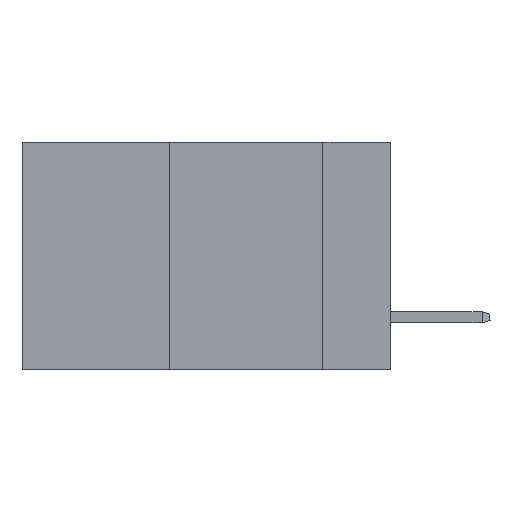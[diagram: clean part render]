
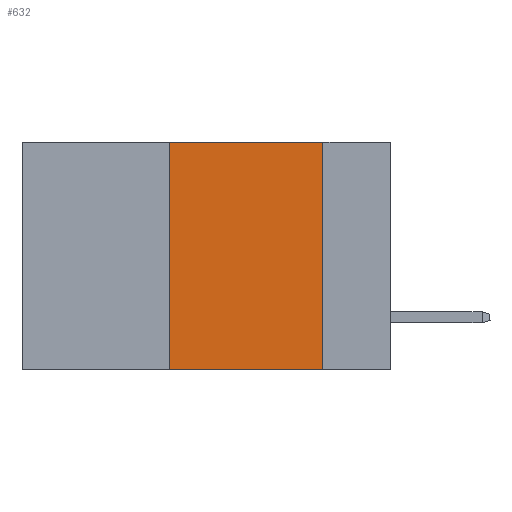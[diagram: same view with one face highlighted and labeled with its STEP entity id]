
A CAD part, left-side view. The second image highlights one B-rep face of the part: STEP entity #632.
In plain terms, the highlighted planar face has unit normal (-1, 0, 0).
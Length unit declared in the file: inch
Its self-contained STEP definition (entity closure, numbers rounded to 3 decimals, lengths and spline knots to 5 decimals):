
#632 = ADVANCED_FACE ( 'NONE', ( #15207 ), #27945, .F. ) ;
#951 = VECTOR ( 'NONE', #22163, 39.37008 ) ;
#1521 = CARTESIAN_POINT ( 'NONE',  ( 0., 0.36, -0.37 ) ) ;
#1534 = DIRECTION ( 'NONE',  ( 0., -1., 0. ) ) ;
#1696 = DIRECTION ( 'NONE',  ( 0., 0., -1. ) ) ;
#2200 = VERTEX_POINT ( 'NONE', #24171 ) ;
#4333 = ORIENTED_EDGE ( 'NONE', *, *, #21173, .F. ) ;
#4380 = LINE ( 'NONE', #22744, #18319 ) ;
#4994 = VERTEX_POINT ( 'NONE', #8363 ) ;
#7084 = LINE ( 'NONE', #18737, #25056 ) ;
#8363 = CARTESIAN_POINT ( 'NONE',  ( 0., 0.11, 0. ) ) ;
#8763 = LINE ( 'NONE', #22068, #951 ) ;
#9481 = EDGE_LOOP ( 'NONE', ( #4333, #19228, #18112, #19227 ) ) ;
#10338 = EDGE_CURVE ( 'NONE', #14017, #14317, #19107, .T. ) ;
#10437 = CARTESIAN_POINT ( 'NONE',  ( 0., 0.6, -0.37 ) ) ;
#12323 = DIRECTION ( 'NONE',  ( 0., -1., 0. ) ) ;
#14017 = VERTEX_POINT ( 'NONE', #1521 ) ;
#14317 = VERTEX_POINT ( 'NONE', #24452 ) ;
#14990 = DIRECTION ( 'NONE',  ( 1., 0., 0. ) ) ;
#15207 = FACE_OUTER_BOUND ( 'NONE', #9481, .T. ) ;
#18112 = ORIENTED_EDGE ( 'NONE', *, *, #21806, .F. ) ;
#18319 = VECTOR ( 'NONE', #1696, 39.37008 ) ;
#18737 = CARTESIAN_POINT ( 'NONE',  ( 0., 0.6, 0. ) ) ;
#19107 = LINE ( 'NONE', #10437, #22087 ) ;
#19227 = ORIENTED_EDGE ( 'NONE', *, *, #10338, .T. ) ;
#19228 = ORIENTED_EDGE ( 'NONE', *, *, #21608, .F. ) ;
#21173 = EDGE_CURVE ( 'NONE', #4994, #14317, #4380, .T. ) ;
#21201 = AXIS2_PLACEMENT_3D ( 'NONE', #25843, #14990, #27763 ) ;
#21608 = EDGE_CURVE ( 'NONE', #2200, #4994, #7084, .T. ) ;
#21806 = EDGE_CURVE ( 'NONE', #14017, #2200, #8763, .T. ) ;
#22068 = CARTESIAN_POINT ( 'NONE',  ( 0., 0.36, 0. ) ) ;
#22087 = VECTOR ( 'NONE', #12323, 39.37008 ) ;
#22163 = DIRECTION ( 'NONE',  ( 0., 0., 1. ) ) ;
#22744 = CARTESIAN_POINT ( 'NONE',  ( 0., 0.11, 0. ) ) ;
#24171 = CARTESIAN_POINT ( 'NONE',  ( 0., 0.36, 0. ) ) ;
#24452 = CARTESIAN_POINT ( 'NONE',  ( 0., 0.11, -0.37 ) ) ;
#25056 = VECTOR ( 'NONE', #1534, 39.37008 ) ;
#25843 = CARTESIAN_POINT ( 'NONE',  ( 0., 0.6, 0. ) ) ;
#27763 = DIRECTION ( 'NONE',  ( 0., 0., -1. ) ) ;
#27945 = PLANE ( 'NONE',  #21201 ) ;
